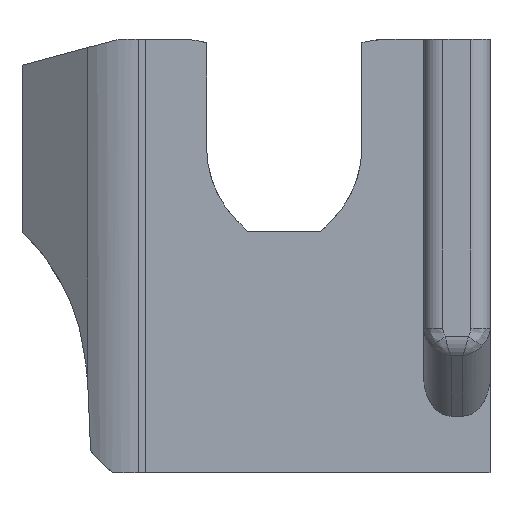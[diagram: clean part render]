
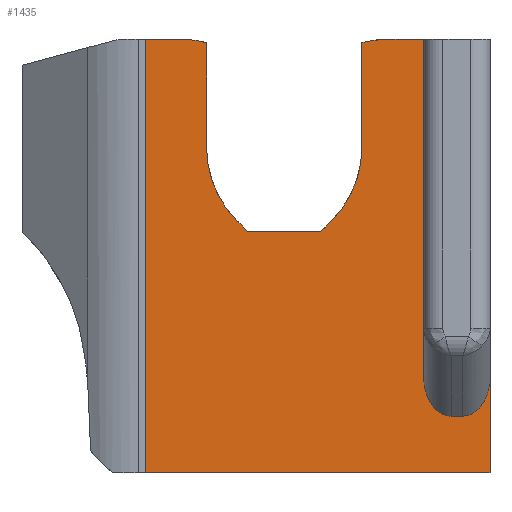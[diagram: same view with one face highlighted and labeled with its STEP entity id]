
A CAD part, left-side view. The second image highlights one B-rep face of the part: STEP entity #1435.
In plain terms, the highlighted planar face has unit normal (-1, 0, 0).
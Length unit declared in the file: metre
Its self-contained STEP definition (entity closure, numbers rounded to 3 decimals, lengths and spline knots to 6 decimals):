
#25=ELLIPSE('',#1544,0.001796,0.00127);
#26=ELLIPSE('',#1545,0.001796,0.00127);
#59=B_SPLINE_CURVE_WITH_KNOTS('',3,(#2191,#2192,#2193,#2194),
 .UNSPECIFIED.,.F.,.F.,(4,4),(0.,0.001117),.UNSPECIFIED.);
#60=B_SPLINE_CURVE_WITH_KNOTS('',3,(#2211,#2212,#2213,#2214),
 .UNSPECIFIED.,.F.,.F.,(4,4),(0.,0.001117),.UNSPECIFIED.);
#80=CIRCLE('',#1543,0.004775);
#81=CIRCLE('',#1546,0.004775);
#165=ORIENTED_EDGE('',*,*,#602,.F.);
#166=ORIENTED_EDGE('',*,*,#603,.T.);
#167=ORIENTED_EDGE('',*,*,#604,.T.);
#168=ORIENTED_EDGE('',*,*,#605,.T.);
#169=ORIENTED_EDGE('',*,*,#606,.T.);
#170=ORIENTED_EDGE('',*,*,#607,.T.);
#171=ORIENTED_EDGE('',*,*,#608,.T.);
#172=ORIENTED_EDGE('',*,*,#609,.F.);
#173=ORIENTED_EDGE('',*,*,#610,.F.);
#174=ORIENTED_EDGE('',*,*,#611,.T.);
#175=ORIENTED_EDGE('',*,*,#612,.F.);
#176=ORIENTED_EDGE('',*,*,#613,.T.);
#177=ORIENTED_EDGE('',*,*,#614,.F.);
#178=ORIENTED_EDGE('',*,*,#574,.T.);
#179=ORIENTED_EDGE('',*,*,#615,.T.);
#180=ORIENTED_EDGE('',*,*,#616,.F.);
#181=ORIENTED_EDGE('',*,*,#617,.T.);
#182=ORIENTED_EDGE('',*,*,#618,.T.);
#574=EDGE_CURVE('',#794,#793,#930,.T.);
#602=EDGE_CURVE('',#820,#821,#949,.T.);
#603=EDGE_CURVE('',#820,#822,#950,.F.);
#604=EDGE_CURVE('',#822,#823,#80,.F.);
#605=EDGE_CURVE('',#823,#824,#951,.T.);
#606=EDGE_CURVE('',#824,#825,#59,.T.);
#607=EDGE_CURVE('',#825,#826,#952,.T.);
#608=EDGE_CURVE('',#826,#827,#953,.T.);
#609=EDGE_CURVE('',#828,#827,#954,.T.);
#610=EDGE_CURVE('',#829,#828,#955,.T.);
#611=EDGE_CURVE('',#829,#830,#25,.F.);
#612=EDGE_CURVE('',#831,#830,#956,.T.);
#613=EDGE_CURVE('',#831,#832,#26,.F.);
#614=EDGE_CURVE('',#794,#832,#957,.T.);
#615=EDGE_CURVE('',#793,#833,#60,.T.);
#616=EDGE_CURVE('',#834,#833,#958,.T.);
#617=EDGE_CURVE('',#834,#835,#81,.F.);
#618=EDGE_CURVE('',#835,#821,#959,.T.);
#793=VERTEX_POINT('',#2119);
#794=VERTEX_POINT('',#2121);
#820=VERTEX_POINT('',#2183);
#821=VERTEX_POINT('',#2184);
#822=VERTEX_POINT('',#2186);
#823=VERTEX_POINT('',#2188);
#824=VERTEX_POINT('',#2190);
#825=VERTEX_POINT('',#2195);
#826=VERTEX_POINT('',#2197);
#827=VERTEX_POINT('',#2199);
#828=VERTEX_POINT('',#2201);
#829=VERTEX_POINT('',#2203);
#830=VERTEX_POINT('',#2205);
#831=VERTEX_POINT('',#2207);
#832=VERTEX_POINT('',#2209);
#833=VERTEX_POINT('',#2215);
#834=VERTEX_POINT('',#2217);
#835=VERTEX_POINT('',#2219);
#930=LINE('',#2120,#1072);
#949=LINE('',#2182,#1091);
#950=LINE('',#2185,#1092);
#951=LINE('',#2189,#1093);
#952=LINE('',#2196,#1094);
#953=LINE('',#2198,#1095);
#954=LINE('',#2200,#1096);
#955=LINE('',#2202,#1097);
#956=LINE('',#2206,#1098);
#957=LINE('',#2210,#1099);
#958=LINE('',#2216,#1100);
#959=LINE('',#2220,#1101);
#1072=VECTOR('',#1693,1.);
#1091=VECTOR('',#1730,1.);
#1092=VECTOR('',#1731,1.);
#1093=VECTOR('',#1734,1.);
#1094=VECTOR('',#1735,1.);
#1095=VECTOR('',#1736,1.);
#1096=VECTOR('',#1737,1.);
#1097=VECTOR('',#1738,1.);
#1098=VECTOR('',#1741,1.);
#1099=VECTOR('',#1744,1.);
#1100=VECTOR('',#1745,1.);
#1101=VECTOR('',#1748,1.);
#1209=EDGE_LOOP('',(#165,#166,#167,#168,#169,#170,#171,#172,#173,#174,#175,
#176,#177,#178,#179,#180,#181,#182));
#1297=FACE_BOUND('',#1209,.T.);
#1383=PLANE('',#1542);
#1435=ADVANCED_FACE('',(#1297),#1383,.T.);
#1542=AXIS2_PLACEMENT_3D('',#2181,#1728,#1729);
#1543=AXIS2_PLACEMENT_3D('',#2187,#1732,#1733);
#1544=AXIS2_PLACEMENT_3D('',#2204,#1739,#1740);
#1545=AXIS2_PLACEMENT_3D('',#2208,#1742,#1743);
#1546=AXIS2_PLACEMENT_3D('',#2218,#1746,#1747);
#1693=DIRECTION('',(0.,1.,0.));
#1728=DIRECTION('',(-1.,0.,0.));
#1729=DIRECTION('',(0.,0.,1.));
#1730=DIRECTION('',(0.,-1.,0.));
#1731=DIRECTION('',(0.,-0.707,-0.707));
#1732=DIRECTION('',(-1.,0.,0.));
#1733=DIRECTION('',(0.,0.,1.));
#1734=DIRECTION('',(0.,0.,1.));
#1735=DIRECTION('',(0.,1.,0.));
#1736=DIRECTION('',(0.,0.,-1.));
#1737=DIRECTION('',(0.,1.,0.));
#1738=DIRECTION('',(0.,0.,-1.));
#1739=DIRECTION('',(-1.,0.,0.));
#1740=DIRECTION('',(0.,0.,-1.));
#1741=DIRECTION('',(0.,-1.,0.));
#1742=DIRECTION('',(-1.,0.,0.));
#1743=DIRECTION('',(0.,0.,1.));
#1744=DIRECTION('',(0.,0.,-1.));
#1745=DIRECTION('',(0.,0.,1.));
#1746=DIRECTION('',(-1.,0.,0.));
#1747=DIRECTION('',(0.,0.,1.));
#1748=DIRECTION('',(0.,0.707,-0.707));
#2119=CARTESIAN_POINT('',(0.002359,0.040645,0.00923));
#2120=CARTESIAN_POINT('',(0.002359,0.045333,0.00923));
#2121=CARTESIAN_POINT('',(0.002359,0.038894,0.00923));
#2181=CARTESIAN_POINT('',(0.002359,0.045333,0.00923));
#2182=CARTESIAN_POINT('',(0.002359,0.045347,0.000341));
#2183=CARTESIAN_POINT('',(0.002359,0.047037,0.000341));
#2184=CARTESIAN_POINT('',(0.002359,0.043657,0.000341));
#2185=CARTESIAN_POINT('',(0.002359,0.047037,0.000341));
#2186=CARTESIAN_POINT('',(0.002359,0.047543,0.000847));
#2187=CARTESIAN_POINT('',(0.002359,0.044167,0.004224));
#2188=CARTESIAN_POINT('',(0.002359,0.048942,0.004224));
#2189=CARTESIAN_POINT('',(0.002359,0.048942,-0.00347));
#2190=CARTESIAN_POINT('',(0.002359,0.048942,0.009078));
#2191=CARTESIAN_POINT('',(0.002359,0.048942,0.009078));
#2192=CARTESIAN_POINT('',(0.002359,0.049305,0.009174));
#2193=CARTESIAN_POINT('',(0.002359,0.049673,0.00923));
#2194=CARTESIAN_POINT('',(0.002359,0.050049,0.00923));
#2195=CARTESIAN_POINT('',(0.002359,0.050049,0.00923));
#2196=CARTESIAN_POINT('',(0.002359,0.045333,0.00923));
#2197=CARTESIAN_POINT('',(0.002359,0.051772,0.00923));
#2198=CARTESIAN_POINT('',(0.002359,0.051772,0.00923));
#2199=CARTESIAN_POINT('',(0.002359,0.051772,-0.01082));
#2200=CARTESIAN_POINT('',(0.002359,0.045333,-0.01082));
#2201=CARTESIAN_POINT('',(0.002359,0.03582,-0.01082));
#2202=CARTESIAN_POINT('',(0.002359,0.03582,-0.009014));
#2203=CARTESIAN_POINT('',(0.002359,0.03582,-0.006411));
#2204=CARTESIAN_POINT('',(0.002359,0.03709,-0.006411));
#2205=CARTESIAN_POINT('',(0.002359,0.03709,-0.008208));
#2206=CARTESIAN_POINT('',(0.002359,0.04217,-0.008208));
#2207=CARTESIAN_POINT('',(0.002359,0.037624,-0.008208));
#2208=CARTESIAN_POINT('',(0.002359,0.037624,-0.006411));
#2209=CARTESIAN_POINT('',(0.002359,0.038894,-0.006411));
#2210=CARTESIAN_POINT('',(0.002359,0.038894,0.00923));
#2211=CARTESIAN_POINT('',(0.002359,0.040645,0.00923));
#2212=CARTESIAN_POINT('',(0.002359,0.041021,0.00923));
#2213=CARTESIAN_POINT('',(0.002359,0.041389,0.009174));
#2214=CARTESIAN_POINT('',(0.002359,0.041752,0.009078));
#2215=CARTESIAN_POINT('',(0.002359,0.041752,0.009078));
#2216=CARTESIAN_POINT('',(0.002359,0.041752,-0.00347));
#2217=CARTESIAN_POINT('',(0.002359,0.041752,0.004224));
#2218=CARTESIAN_POINT('',(0.002359,0.046527,0.004224));
#2219=CARTESIAN_POINT('',(0.002359,0.043151,0.000847));
#2220=CARTESIAN_POINT('',(0.002359,0.041752,0.002246));
